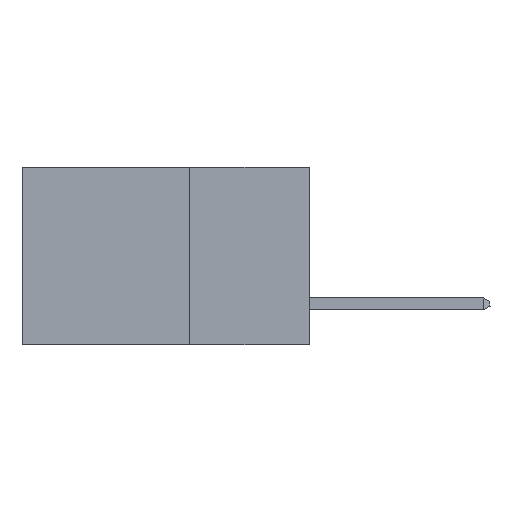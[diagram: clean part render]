
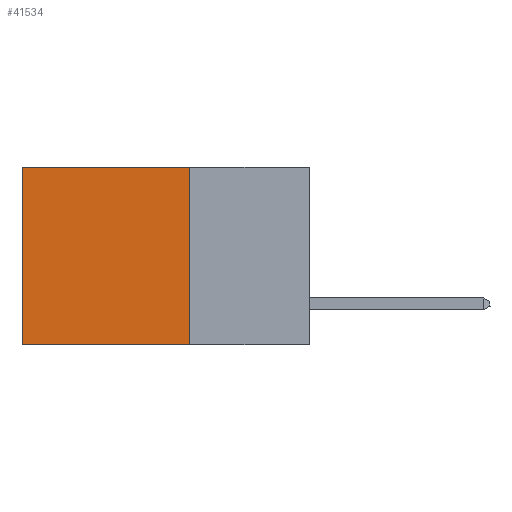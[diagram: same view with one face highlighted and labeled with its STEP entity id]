
A CAD part, left-side view. The second image highlights one B-rep face of the part: STEP entity #41534.
In plain terms, the highlighted planar face has unit normal (-1, 0, 0).
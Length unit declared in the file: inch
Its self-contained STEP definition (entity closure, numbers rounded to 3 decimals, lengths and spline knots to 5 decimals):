
#242 = VERTEX_POINT ( 'NONE', #3377 ) ;
#1423 = VECTOR ( 'NONE', #7778, 39.37008 ) ;
#3377 = CARTESIAN_POINT ( 'NONE',  ( 0.2875, 0.25, -0.37 ) ) ;
#3940 = LINE ( 'NONE', #8895, #23625 ) ;
#5631 = EDGE_CURVE ( 'NONE', #19964, #20662, #33769, .T. ) ;
#7778 = DIRECTION ( 'NONE',  ( 0., 0., -1. ) ) ;
#8451 = ORIENTED_EDGE ( 'NONE', *, *, #19873, .F. ) ;
#8895 = CARTESIAN_POINT ( 'NONE',  ( 0.2875, 0.25, -0.37 ) ) ;
#10645 = EDGE_CURVE ( 'NONE', #38740, #19964, #15841, .T. ) ;
#12027 = DIRECTION ( 'NONE',  ( 1., 0., 0. ) ) ;
#12215 = CARTESIAN_POINT ( 'NONE',  ( 0.2875, 0.6, 0. ) ) ;
#13493 = CARTESIAN_POINT ( 'NONE',  ( 0.2875, 0.6, 0. ) ) ;
#15729 = PLANE ( 'NONE',  #24979 ) ;
#15758 = CARTESIAN_POINT ( 'NONE',  ( 0.2875, 0.6, -0.37 ) ) ;
#15841 = LINE ( 'NONE', #17622, #48170 ) ;
#16831 = ORIENTED_EDGE ( 'NONE', *, *, #10645, .T. ) ;
#17622 = CARTESIAN_POINT ( 'NONE',  ( 0.2875, 0.25, 0. ) ) ;
#19873 = EDGE_CURVE ( 'NONE', #242, #20662, #3940, .T. ) ;
#19964 = VERTEX_POINT ( 'NONE', #13493 ) ;
#20019 = VECTOR ( 'NONE', #45026, 39.37008 ) ;
#20662 = VERTEX_POINT ( 'NONE', #15758 ) ;
#23035 = LINE ( 'NONE', #41193, #20019 ) ;
#23625 = VECTOR ( 'NONE', #35926, 39.37008 ) ;
#24979 = AXIS2_PLACEMENT_3D ( 'NONE', #31439, #12027, #34951 ) ;
#27967 = EDGE_LOOP ( 'NONE', ( #45652, #8451, #40317, #16831 ) ) ;
#30394 = FACE_OUTER_BOUND ( 'NONE', #27967, .T. ) ;
#30845 = CARTESIAN_POINT ( 'NONE',  ( 0.2875, 0.25, 0. ) ) ;
#31439 = CARTESIAN_POINT ( 'NONE',  ( 0.2875, 0.25, 0. ) ) ;
#32233 = DIRECTION ( 'NONE',  ( 0., 1., 0. ) ) ;
#33769 = LINE ( 'NONE', #12215, #1423 ) ;
#34951 = DIRECTION ( 'NONE',  ( 0., 0., -1. ) ) ;
#35926 = DIRECTION ( 'NONE',  ( 0., 1., 0. ) ) ;
#38740 = VERTEX_POINT ( 'NONE', #30845 ) ;
#40317 = ORIENTED_EDGE ( 'NONE', *, *, #42658, .F. ) ;
#41193 = CARTESIAN_POINT ( 'NONE',  ( 0.2875, 0.25, 0. ) ) ;
#41534 = ADVANCED_FACE ( 'NONE', ( #30394 ), #15729, .F. ) ;
#42658 = EDGE_CURVE ( 'NONE', #38740, #242, #23035, .T. ) ;
#45026 = DIRECTION ( 'NONE',  ( 0., 0., -1. ) ) ;
#45652 = ORIENTED_EDGE ( 'NONE', *, *, #5631, .T. ) ;
#48170 = VECTOR ( 'NONE', #32233, 39.37008 ) ;
